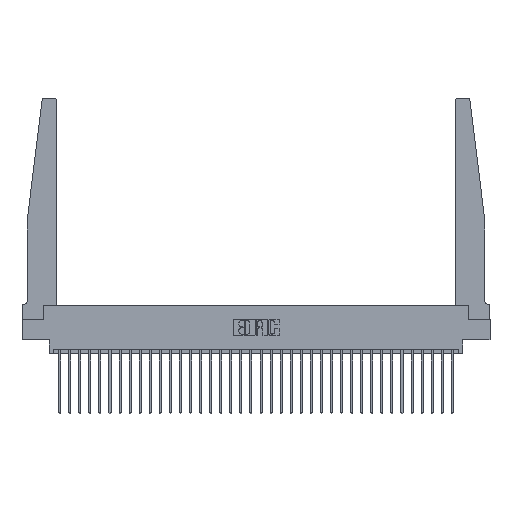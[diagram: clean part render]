
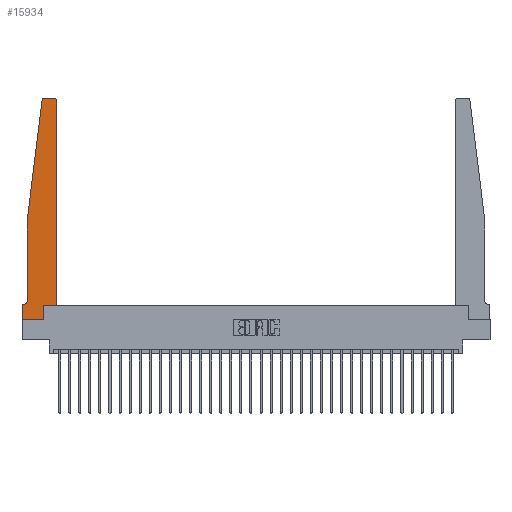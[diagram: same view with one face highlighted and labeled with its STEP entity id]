
A CAD part, top view. The second image highlights one B-rep face of the part: STEP entity #15934.
In plain terms, the highlighted planar face has unit normal (0, 0, 1).
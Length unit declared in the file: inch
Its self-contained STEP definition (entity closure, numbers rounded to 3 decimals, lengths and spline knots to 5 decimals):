
#383 = ORIENTED_EDGE ( 'NONE', *, *, #28676, .T. ) ;
#507 = VECTOR ( 'NONE', #21645, 39.37008 ) ;
#891 = CARTESIAN_POINT ( 'NONE',  ( 0.015, 0.2375, 0.37 ) ) ;
#1352 = VECTOR ( 'NONE', #21734, 39.37008 ) ;
#1723 = DIRECTION ( 'NONE',  ( 1., 0., 0. ) ) ;
#1786 = EDGE_CURVE ( 'NONE', #21706, #19821, #26296, .T. ) ;
#2190 = ORIENTED_EDGE ( 'NONE', *, *, #29559, .T. ) ;
#2393 = CARTESIAN_POINT ( 'NONE',  ( 0., 0., 0.37 ) ) ;
#2507 = LINE ( 'NONE', #7591, #13840 ) ;
#2705 = DIRECTION ( 'NONE',  ( 0., -1., 0. ) ) ;
#3317 = DIRECTION ( 'NONE',  ( -1., 0., 0. ) ) ;
#3345 = VERTEX_POINT ( 'NONE', #22231 ) ;
#3493 = CARTESIAN_POINT ( 'NONE',  ( 0.015, 0.1875, 0.37 ) ) ;
#4188 = ORIENTED_EDGE ( 'NONE', *, *, #25277, .T. ) ;
#4785 = DIRECTION ( 'NONE',  ( 0., 0., 1. ) ) ;
#4899 = LINE ( 'NONE', #23180, #30641 ) ;
#5205 = DIRECTION ( 'NONE',  ( 0., 0., 1. ) ) ;
#5519 = EDGE_CURVE ( 'NONE', #16986, #14588, #8774, .T. ) ;
#5520 = LINE ( 'NONE', #19960, #11926 ) ;
#6942 = LINE ( 'NONE', #9519, #507 ) ;
#7116 = PLANE ( 'NONE',  #19923 ) ;
#7591 = CARTESIAN_POINT ( 'NONE',  ( 0.065, 1.25, 0.37 ) ) ;
#7784 = CIRCLE ( 'NONE', #15275, 0.05 ) ;
#7929 = CIRCLE ( 'NONE', #12854, 0.03 ) ;
#8704 = DIRECTION ( 'NONE',  ( 0., 1., 0. ) ) ;
#8774 = LINE ( 'NONE', #16383, #28068 ) ;
#9336 = VERTEX_POINT ( 'NONE', #24872 ) ;
#9519 = CARTESIAN_POINT ( 'NONE',  ( 0.25, 2.75, 0.37 ) ) ;
#9929 = CARTESIAN_POINT ( 'NONE',  ( 0.395, 2.72, 0.37 ) ) ;
#10326 = CIRCLE ( 'NONE', #14107, 0.03 ) ;
#10831 = CARTESIAN_POINT ( 'NONE',  ( 0.065, 0.2375, 0.37 ) ) ;
#11427 = ORIENTED_EDGE ( 'NONE', *, *, #24908, .T. ) ;
#11524 = EDGE_CURVE ( 'NONE', #19821, #17860, #2507, .T. ) ;
#11817 = CARTESIAN_POINT ( 'NONE',  ( 0., 0., 0.37 ) ) ;
#11837 = DIRECTION ( 'NONE',  ( -1., 0., 0. ) ) ;
#11892 = CARTESIAN_POINT ( 'NONE',  ( 0.2605, 0., 0.37 ) ) ;
#11926 = VECTOR ( 'NONE', #15118, 39.37008 ) ;
#11959 = CARTESIAN_POINT ( 'NONE',  ( 0., 0.1875, 0.37 ) ) ;
#12234 = EDGE_CURVE ( 'NONE', #17860, #22405, #7784, .T. ) ;
#12353 = DIRECTION ( 'NONE',  ( 1., 0., 0. ) ) ;
#12501 = CARTESIAN_POINT ( 'NONE',  ( 0., 0., 0.37 ) ) ;
#12854 = AXIS2_PLACEMENT_3D ( 'NONE', #9929, #26851, #12353 ) ;
#12927 = ORIENTED_EDGE ( 'NONE', *, *, #23478, .T. ) ;
#13840 = VECTOR ( 'NONE', #2705, 39.37008 ) ;
#14107 = AXIS2_PLACEMENT_3D ( 'NONE', #19623, #5205, #22087 ) ;
#14261 = LINE ( 'NONE', #23899, #27950 ) ;
#14421 = ORIENTED_EDGE ( 'NONE', *, *, #5519, .T. ) ;
#14588 = VERTEX_POINT ( 'NONE', #26208 ) ;
#15118 = DIRECTION ( 'NONE',  ( 0., 1., 0. ) ) ;
#15170 = VERTEX_POINT ( 'NONE', #23338 ) ;
#15275 = AXIS2_PLACEMENT_3D ( 'NONE', #891, #17756, #3317 ) ;
#15335 = VERTEX_POINT ( 'NONE', #11892 ) ;
#15934 = ADVANCED_FACE ( 'NONE', ( #24176 ), #7116, .T. ) ;
#16383 = CARTESIAN_POINT ( 'NONE',  ( 0.425, 0.18, 0.37 ) ) ;
#16958 = CARTESIAN_POINT ( 'NONE',  ( 0.065, 1.25, 0.37 ) ) ;
#16986 = VERTEX_POINT ( 'NONE', #18119 ) ;
#17756 = DIRECTION ( 'NONE',  ( 0., 0., -1. ) ) ;
#17860 = VERTEX_POINT ( 'NONE', #10831 ) ;
#18119 = CARTESIAN_POINT ( 'NONE',  ( 0.2605, 0.18, 0.37 ) ) ;
#18238 = ORIENTED_EDGE ( 'NONE', *, *, #11524, .T. ) ;
#18315 = EDGE_CURVE ( 'NONE', #3345, #21706, #10326, .T. ) ;
#19398 = ORIENTED_EDGE ( 'NONE', *, *, #21998, .T. ) ;
#19623 = CARTESIAN_POINT ( 'NONE',  ( 0.27653, 2.72, 0.37 ) ) ;
#19821 = VERTEX_POINT ( 'NONE', #27987 ) ;
#19923 = AXIS2_PLACEMENT_3D ( 'NONE', #11959, #4785, #21666 ) ;
#19960 = CARTESIAN_POINT ( 'NONE',  ( 0.2605, 0.18, 0.37 ) ) ;
#20269 = VECTOR ( 'NONE', #29452, 39.37008 ) ;
#21029 = LINE ( 'NONE', #12501, #20269 ) ;
#21645 = DIRECTION ( 'NONE',  ( -1., 0., 0. ) ) ;
#21666 = DIRECTION ( 'NONE',  ( 1., 0., 0. ) ) ;
#21706 = VERTEX_POINT ( 'NONE', #27843 ) ;
#21734 = DIRECTION ( 'NONE',  ( -0.122, -0.992, 0. ) ) ;
#21998 = EDGE_CURVE ( 'NONE', #22405, #23423, #14261, .T. ) ;
#22087 = DIRECTION ( 'NONE',  ( 1., 0., 0. ) ) ;
#22231 = CARTESIAN_POINT ( 'NONE',  ( 0.27653, 2.75, 0.37 ) ) ;
#22405 = VERTEX_POINT ( 'NONE', #3493 ) ;
#22775 = LINE ( 'NONE', #11817, #29227 ) ;
#23180 = CARTESIAN_POINT ( 'NONE',  ( 0.425, 0.18, 0.37 ) ) ;
#23338 = CARTESIAN_POINT ( 'NONE',  ( 0.425, 2.72, 0.37 ) ) ;
#23423 = VERTEX_POINT ( 'NONE', #24559 ) ;
#23478 = EDGE_CURVE ( 'NONE', #15335, #16986, #5520, .T. ) ;
#23899 = CARTESIAN_POINT ( 'NONE',  ( 0.065, 0.1875, 0.37 ) ) ;
#24038 = VERTEX_POINT ( 'NONE', #2393 ) ;
#24176 = FACE_OUTER_BOUND ( 'NONE', #26026, .T. ) ;
#24559 = CARTESIAN_POINT ( 'NONE',  ( 0., 0.1875, 0.37 ) ) ;
#24872 = CARTESIAN_POINT ( 'NONE',  ( 0.395, 2.75, 0.37 ) ) ;
#24908 = EDGE_CURVE ( 'NONE', #14588, #15170, #4899, .T. ) ;
#25277 = EDGE_CURVE ( 'NONE', #15170, #9336, #7929, .T. ) ;
#26026 = EDGE_LOOP ( 'NONE', ( #383, #27801, #30585, #18238, #27430, #19398, #2190, #30810, #12927, #14421, #11427, #4188 ) ) ;
#26208 = CARTESIAN_POINT ( 'NONE',  ( 0.425, 0.18, 0.37 ) ) ;
#26296 = LINE ( 'NONE', #16958, #1352 ) ;
#26463 = EDGE_CURVE ( 'NONE', #24038, #15335, #21029, .T. ) ;
#26851 = DIRECTION ( 'NONE',  ( 0., 0., 1. ) ) ;
#27430 = ORIENTED_EDGE ( 'NONE', *, *, #12234, .T. ) ;
#27801 = ORIENTED_EDGE ( 'NONE', *, *, #18315, .T. ) ;
#27843 = CARTESIAN_POINT ( 'NONE',  ( 0.24675, 2.72367, 0.37 ) ) ;
#27950 = VECTOR ( 'NONE', #11837, 39.37008 ) ;
#27987 = CARTESIAN_POINT ( 'NONE',  ( 0.065, 1.25, 0.37 ) ) ;
#28068 = VECTOR ( 'NONE', #1723, 39.37008 ) ;
#28676 = EDGE_CURVE ( 'NONE', #9336, #3345, #6942, .T. ) ;
#28760 = DIRECTION ( 'NONE',  ( 0., -1., 0. ) ) ;
#29227 = VECTOR ( 'NONE', #28760, 39.37008 ) ;
#29452 = DIRECTION ( 'NONE',  ( 1., 0., 0. ) ) ;
#29559 = EDGE_CURVE ( 'NONE', #23423, #24038, #22775, .T. ) ;
#30585 = ORIENTED_EDGE ( 'NONE', *, *, #1786, .T. ) ;
#30641 = VECTOR ( 'NONE', #8704, 39.37008 ) ;
#30810 = ORIENTED_EDGE ( 'NONE', *, *, #26463, .T. ) ;
